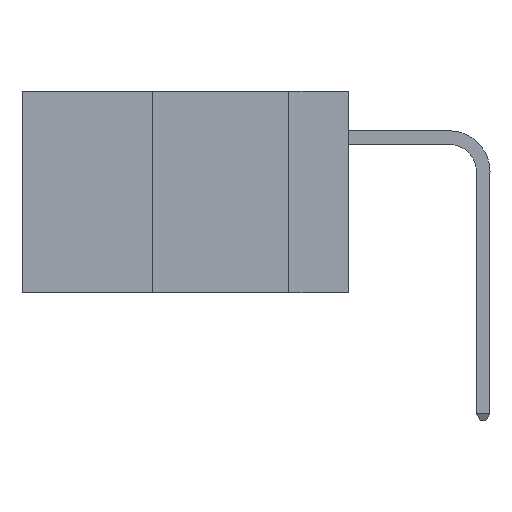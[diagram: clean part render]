
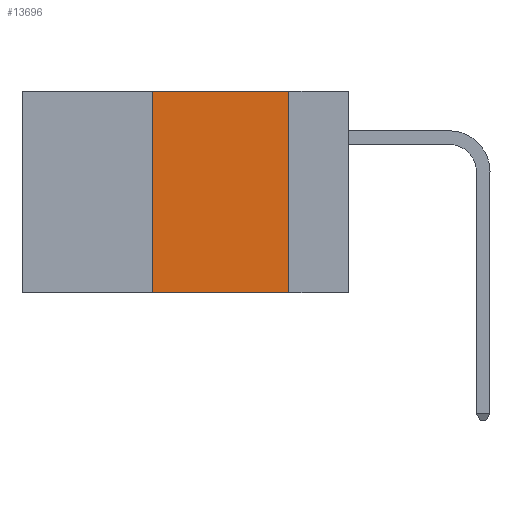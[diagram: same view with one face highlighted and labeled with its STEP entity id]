
A CAD part, left-side view. The second image highlights one B-rep face of the part: STEP entity #13696.
In plain terms, the highlighted planar face has unit normal (-1, 0, 0).
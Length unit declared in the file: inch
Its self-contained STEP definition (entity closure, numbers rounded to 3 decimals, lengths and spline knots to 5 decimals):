
#23 = VECTOR ( 'NONE', #58, 39.37008 ) ;
#58 = DIRECTION ( 'NONE',  ( 0., -1., 0. ) ) ;
#440 = VERTEX_POINT ( 'NONE', #3287 ) ;
#593 = EDGE_CURVE ( 'NONE', #8252, #14131, #3331, .T. ) ;
#742 = LINE ( 'NONE', #13450, #10668 ) ;
#1266 = CARTESIAN_POINT ( 'NONE',  ( 0., 0.11, 0. ) ) ;
#2183 = ORIENTED_EDGE ( 'NONE', *, *, #9791, .F. ) ;
#2460 = ORIENTED_EDGE ( 'NONE', *, *, #9036, .T. ) ;
#3287 = CARTESIAN_POINT ( 'NONE',  ( 0., 0.36, 0. ) ) ;
#3331 = LINE ( 'NONE', #1266, #14290 ) ;
#4076 = DIRECTION ( 'NONE',  ( 0., -1., 0. ) ) ;
#4307 = FACE_OUTER_BOUND ( 'NONE', #8633, .T. ) ;
#4496 = EDGE_CURVE ( 'NONE', #440, #8252, #9204, .T. ) ;
#4790 = AXIS2_PLACEMENT_3D ( 'NONE', #8187, #12689, #8083 ) ;
#5699 = CARTESIAN_POINT ( 'NONE',  ( 0., 0.36, -0.37 ) ) ;
#5925 = CARTESIAN_POINT ( 'NONE',  ( 0., 0.11, 0. ) ) ;
#7431 = CARTESIAN_POINT ( 'NONE',  ( 0., 0.11, -0.37 ) ) ;
#8083 = DIRECTION ( 'NONE',  ( 0., 0., -1. ) ) ;
#8187 = CARTESIAN_POINT ( 'NONE',  ( 0., 0.6, 0. ) ) ;
#8252 = VERTEX_POINT ( 'NONE', #5925 ) ;
#8633 = EDGE_LOOP ( 'NONE', ( #12290, #12548, #2183, #2460 ) ) ;
#9036 = EDGE_CURVE ( 'NONE', #10994, #14131, #10889, .T. ) ;
#9187 = PLANE ( 'NONE',  #4790 ) ;
#9204 = LINE ( 'NONE', #10477, #23 ) ;
#9764 = CARTESIAN_POINT ( 'NONE',  ( 0., 0.6, -0.37 ) ) ;
#9791 = EDGE_CURVE ( 'NONE', #10994, #440, #742, .T. ) ;
#9982 = VECTOR ( 'NONE', #4076, 39.37008 ) ;
#10127 = DIRECTION ( 'NONE',  ( 0., 0., 1. ) ) ;
#10477 = CARTESIAN_POINT ( 'NONE',  ( 0., 0.6, 0. ) ) ;
#10626 = DIRECTION ( 'NONE',  ( 0., 0., -1. ) ) ;
#10668 = VECTOR ( 'NONE', #10127, 39.37008 ) ;
#10889 = LINE ( 'NONE', #9764, #9982 ) ;
#10994 = VERTEX_POINT ( 'NONE', #5699 ) ;
#12290 = ORIENTED_EDGE ( 'NONE', *, *, #593, .F. ) ;
#12548 = ORIENTED_EDGE ( 'NONE', *, *, #4496, .F. ) ;
#12689 = DIRECTION ( 'NONE',  ( 1., 0., 0. ) ) ;
#13450 = CARTESIAN_POINT ( 'NONE',  ( 0., 0.36, 0. ) ) ;
#13696 = ADVANCED_FACE ( 'NONE', ( #4307 ), #9187, .F. ) ;
#14131 = VERTEX_POINT ( 'NONE', #7431 ) ;
#14290 = VECTOR ( 'NONE', #10626, 39.37008 ) ;
